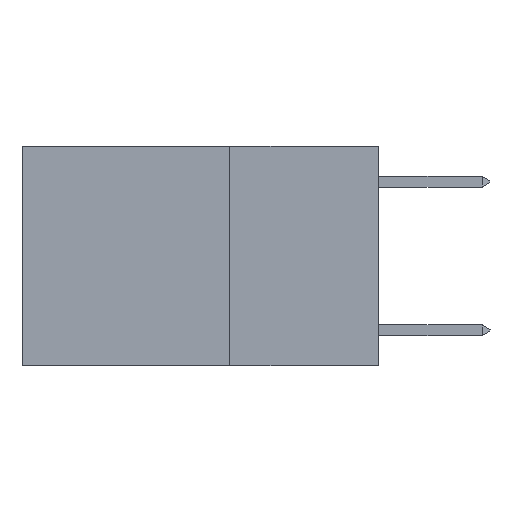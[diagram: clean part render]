
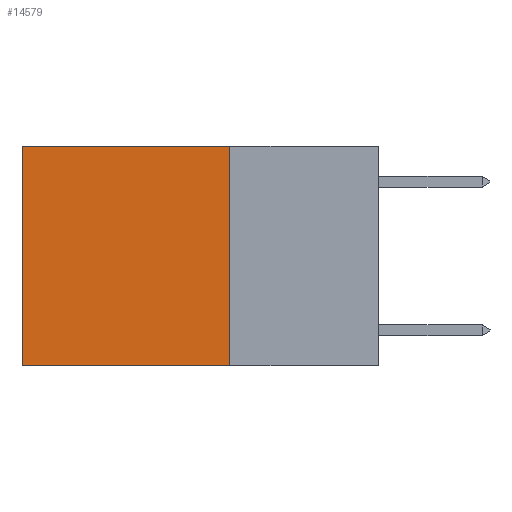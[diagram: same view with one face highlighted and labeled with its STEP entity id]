
A CAD part, left-side view. The second image highlights one B-rep face of the part: STEP entity #14579.
In plain terms, the highlighted planar face has unit normal (-1, 0, 0).
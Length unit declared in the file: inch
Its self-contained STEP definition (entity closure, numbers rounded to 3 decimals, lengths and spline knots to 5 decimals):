
#551 = CARTESIAN_POINT ( 'NONE',  ( 0.2625, 0.25, -0.37 ) ) ;
#791 = VERTEX_POINT ( 'NONE', #14462 ) ;
#1560 = VERTEX_POINT ( 'NONE', #2996 ) ;
#1755 = LINE ( 'NONE', #14521, #10656 ) ;
#1811 = DIRECTION ( 'NONE',  ( 0., 1., 0. ) ) ;
#1825 = CARTESIAN_POINT ( 'NONE',  ( 0.2625, 0.25, 0. ) ) ;
#2029 = VECTOR ( 'NONE', #2327, 39.37008 ) ;
#2327 = DIRECTION ( 'NONE',  ( 0., 0., -1. ) ) ;
#2894 = DIRECTION ( 'NONE',  ( 0., 1., 0. ) ) ;
#2996 = CARTESIAN_POINT ( 'NONE',  ( 0.2625, 0.6, -0.37 ) ) ;
#3093 = DIRECTION ( 'NONE',  ( 0., 0., -1. ) ) ;
#3881 = LINE ( 'NONE', #8366, #14443 ) ;
#4101 = EDGE_CURVE ( 'NONE', #6627, #791, #3881, .T. ) ;
#4714 = CARTESIAN_POINT ( 'NONE',  ( 0.2625, 0.6, 0. ) ) ;
#4789 = LINE ( 'NONE', #551, #11477 ) ;
#6085 = LINE ( 'NONE', #4714, #2029 ) ;
#6627 = VERTEX_POINT ( 'NONE', #12885 ) ;
#6740 = EDGE_CURVE ( 'NONE', #6627, #13005, #1755, .T. ) ;
#6839 = EDGE_LOOP ( 'NONE', ( #13015, #13115, #14934, #11871 ) ) ;
#6986 = EDGE_CURVE ( 'NONE', #791, #1560, #4789, .T. ) ;
#7908 = CARTESIAN_POINT ( 'NONE',  ( 0.2625, 0.6, 0. ) ) ;
#8366 = CARTESIAN_POINT ( 'NONE',  ( 0.2625, 0.25, 0. ) ) ;
#9719 = DIRECTION ( 'NONE',  ( 0., 0., -1. ) ) ;
#9898 = EDGE_CURVE ( 'NONE', #13005, #1560, #6085, .T. ) ;
#10656 = VECTOR ( 'NONE', #2894, 39.37008 ) ;
#11477 = VECTOR ( 'NONE', #1811, 39.37008 ) ;
#11871 = ORIENTED_EDGE ( 'NONE', *, *, #6740, .T. ) ;
#11899 = PLANE ( 'NONE',  #15695 ) ;
#12885 = CARTESIAN_POINT ( 'NONE',  ( 0.2625, 0.25, 0. ) ) ;
#13005 = VERTEX_POINT ( 'NONE', #7908 ) ;
#13015 = ORIENTED_EDGE ( 'NONE', *, *, #9898, .T. ) ;
#13115 = ORIENTED_EDGE ( 'NONE', *, *, #6986, .F. ) ;
#13435 = FACE_OUTER_BOUND ( 'NONE', #6839, .T. ) ;
#13465 = DIRECTION ( 'NONE',  ( 1., 0., 0. ) ) ;
#14443 = VECTOR ( 'NONE', #3093, 39.37008 ) ;
#14462 = CARTESIAN_POINT ( 'NONE',  ( 0.2625, 0.25, -0.37 ) ) ;
#14521 = CARTESIAN_POINT ( 'NONE',  ( 0.2625, 0.25, 0. ) ) ;
#14579 = ADVANCED_FACE ( 'NONE', ( #13435 ), #11899, .F. ) ;
#14934 = ORIENTED_EDGE ( 'NONE', *, *, #4101, .F. ) ;
#15695 = AXIS2_PLACEMENT_3D ( 'NONE', #1825, #13465, #9719 ) ;
